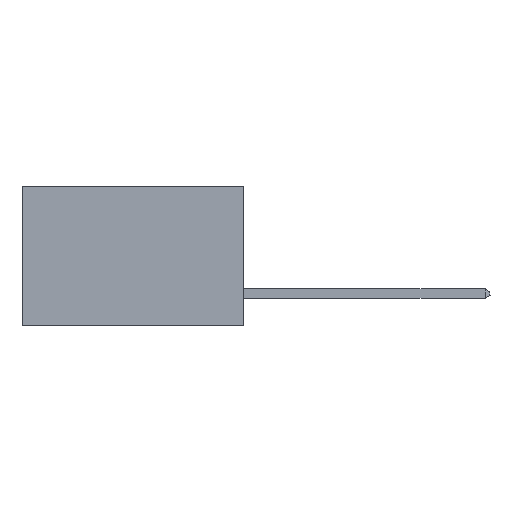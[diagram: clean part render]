
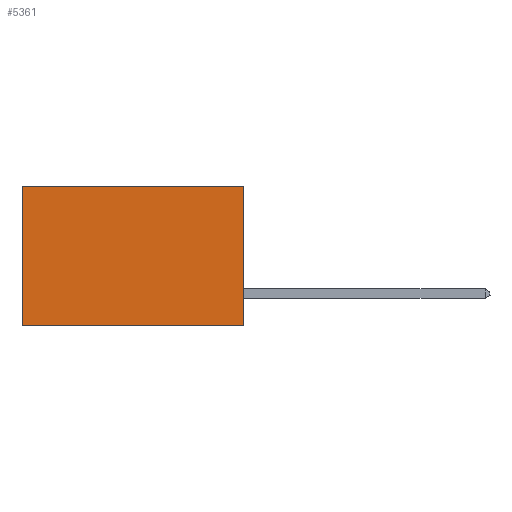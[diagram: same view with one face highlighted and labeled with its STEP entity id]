
A CAD part, left-side view. The second image highlights one B-rep face of the part: STEP entity #5361.
In plain terms, the highlighted planar face has unit normal (-1, 0, 0).
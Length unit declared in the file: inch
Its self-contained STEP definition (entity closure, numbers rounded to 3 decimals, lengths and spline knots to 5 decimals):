
#254 = ORIENTED_EDGE ( 'NONE', *, *, #14040, .T. ) ;
#316 = LINE ( 'NONE', #12785, #7254 ) ;
#839 = VERTEX_POINT ( 'NONE', #10028 ) ;
#1386 = LINE ( 'NONE', #13114, #12637 ) ;
#1652 = VERTEX_POINT ( 'NONE', #3865 ) ;
#2704 = LINE ( 'NONE', #2846, #8622 ) ;
#2846 = CARTESIAN_POINT ( 'NONE',  ( 0.277, 0., -0.37 ) ) ;
#3065 = DIRECTION ( 'NONE',  ( 0., 1., 0. ) ) ;
#3865 = CARTESIAN_POINT ( 'NONE',  ( 0.277, 0.59, 0. ) ) ;
#4644 = EDGE_CURVE ( 'NONE', #10113, #7883, #1386, .T. ) ;
#5034 = CARTESIAN_POINT ( 'NONE',  ( 0.277, 0., -0.37 ) ) ;
#5361 = ADVANCED_FACE ( 'NONE', ( #6799 ), #10007, .F. ) ;
#5625 = EDGE_CURVE ( 'NONE', #1652, #839, #8851, .T. ) ;
#6401 = DIRECTION ( 'NONE',  ( 0., 1., 0. ) ) ;
#6799 = FACE_OUTER_BOUND ( 'NONE', #7583, .T. ) ;
#7254 = VECTOR ( 'NONE', #6401, 39.37008 ) ;
#7571 = ORIENTED_EDGE ( 'NONE', *, *, #5625, .T. ) ;
#7583 = EDGE_LOOP ( 'NONE', ( #7571, #9294, #8431, #254 ) ) ;
#7637 = EDGE_CURVE ( 'NONE', #7883, #839, #2704, .T. ) ;
#7883 = VERTEX_POINT ( 'NONE', #5034 ) ;
#7909 = DIRECTION ( 'NONE',  ( 0., 0., -1. ) ) ;
#8323 = CARTESIAN_POINT ( 'NONE',  ( 0.277, 0.59, -0.37 ) ) ;
#8431 = ORIENTED_EDGE ( 'NONE', *, *, #4644, .F. ) ;
#8622 = VECTOR ( 'NONE', #3065, 39.37008 ) ;
#8851 = LINE ( 'NONE', #8323, #14083 ) ;
#9294 = ORIENTED_EDGE ( 'NONE', *, *, #7637, .F. ) ;
#9411 = DIRECTION ( 'NONE',  ( 0., 0., -1. ) ) ;
#9431 = DIRECTION ( 'NONE',  ( 1., 0., 0. ) ) ;
#9476 = CARTESIAN_POINT ( 'NONE',  ( 0.277, 0., -0.37 ) ) ;
#10007 = PLANE ( 'NONE',  #13129 ) ;
#10028 = CARTESIAN_POINT ( 'NONE',  ( 0.277, 0.59, -0.37 ) ) ;
#10113 = VERTEX_POINT ( 'NONE', #12550 ) ;
#11914 = DIRECTION ( 'NONE',  ( 0., 0., -1. ) ) ;
#12550 = CARTESIAN_POINT ( 'NONE',  ( 0.277, 0., 0. ) ) ;
#12637 = VECTOR ( 'NONE', #11914, 39.37008 ) ;
#12785 = CARTESIAN_POINT ( 'NONE',  ( 0.277, 0., 0. ) ) ;
#13114 = CARTESIAN_POINT ( 'NONE',  ( 0.277, 0., -0.37 ) ) ;
#13129 = AXIS2_PLACEMENT_3D ( 'NONE', #9476, #9431, #9411 ) ;
#14040 = EDGE_CURVE ( 'NONE', #10113, #1652, #316, .T. ) ;
#14083 = VECTOR ( 'NONE', #7909, 39.37008 ) ;
